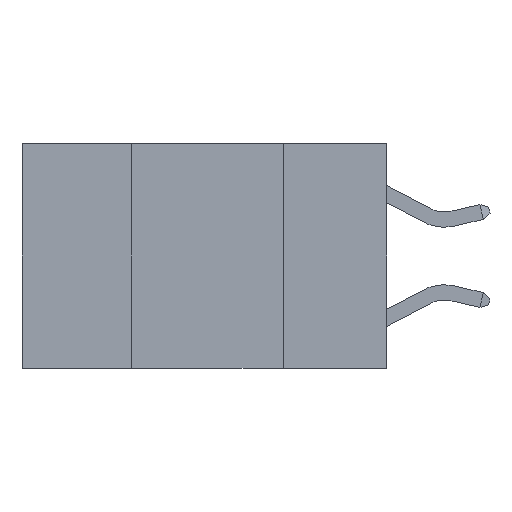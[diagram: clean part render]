
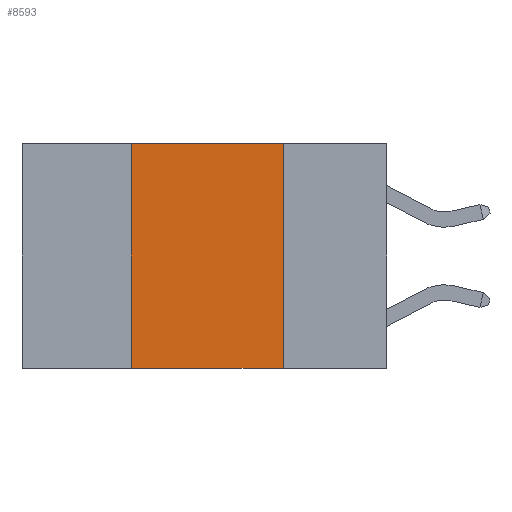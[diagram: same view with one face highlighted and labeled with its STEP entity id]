
A CAD part, left-side view. The second image highlights one B-rep face of the part: STEP entity #8593.
In plain terms, the highlighted planar face has unit normal (-1, 0, 0).
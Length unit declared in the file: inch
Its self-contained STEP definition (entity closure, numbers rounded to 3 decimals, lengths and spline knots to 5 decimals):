
#255 = VECTOR ( 'NONE', #6862, 39.37008 ) ;
#387 = VERTEX_POINT ( 'NONE', #7089 ) ;
#912 = EDGE_CURVE ( 'NONE', #1188, #9660, #5066, .T. ) ;
#1188 = VERTEX_POINT ( 'NONE', #4482 ) ;
#1473 = DIRECTION ( 'NONE',  ( 1., 0., 0. ) ) ;
#2008 = EDGE_CURVE ( 'NONE', #1188, #387, #6338, .T. ) ;
#2725 = VERTEX_POINT ( 'NONE', #5043 ) ;
#2930 = ORIENTED_EDGE ( 'NONE', *, *, #2008, .T. ) ;
#3427 = EDGE_CURVE ( 'NONE', #2725, #387, #4746, .T. ) ;
#3689 = LINE ( 'NONE', #4263, #4199 ) ;
#3884 = AXIS2_PLACEMENT_3D ( 'NONE', #6503, #1473, #7309 ) ;
#4199 = VECTOR ( 'NONE', #9939, 39.37008 ) ;
#4263 = CARTESIAN_POINT ( 'NONE',  ( 0., 0.6, 0. ) ) ;
#4283 = FACE_OUTER_BOUND ( 'NONE', #7953, .T. ) ;
#4482 = CARTESIAN_POINT ( 'NONE',  ( 0., 0.42, -0.37 ) ) ;
#4746 = LINE ( 'NONE', #7647, #255 ) ;
#5043 = CARTESIAN_POINT ( 'NONE',  ( 0., 0.17, 0. ) ) ;
#5066 = LINE ( 'NONE', #9829, #6742 ) ;
#5338 = ORIENTED_EDGE ( 'NONE', *, *, #912, .F. ) ;
#5722 = EDGE_CURVE ( 'NONE', #9660, #2725, #3689, .T. ) ;
#6338 = LINE ( 'NONE', #7128, #10356 ) ;
#6503 = CARTESIAN_POINT ( 'NONE',  ( 0., 0.6, 0. ) ) ;
#6742 = VECTOR ( 'NONE', #9778, 39.37008 ) ;
#6845 = ORIENTED_EDGE ( 'NONE', *, *, #5722, .F. ) ;
#6862 = DIRECTION ( 'NONE',  ( 0., 0., -1. ) ) ;
#7089 = CARTESIAN_POINT ( 'NONE',  ( 0., 0.17, -0.37 ) ) ;
#7128 = CARTESIAN_POINT ( 'NONE',  ( 0., 0.6, -0.37 ) ) ;
#7274 = PLANE ( 'NONE',  #3884 ) ;
#7309 = DIRECTION ( 'NONE',  ( 0., 0., -1. ) ) ;
#7351 = DIRECTION ( 'NONE',  ( 0., -1., 0. ) ) ;
#7647 = CARTESIAN_POINT ( 'NONE',  ( 0., 0.17, 0. ) ) ;
#7704 = CARTESIAN_POINT ( 'NONE',  ( 0., 0.42, 0. ) ) ;
#7953 = EDGE_LOOP ( 'NONE', ( #10040, #6845, #5338, #2930 ) ) ;
#8593 = ADVANCED_FACE ( 'NONE', ( #4283 ), #7274, .F. ) ;
#9660 = VERTEX_POINT ( 'NONE', #7704 ) ;
#9778 = DIRECTION ( 'NONE',  ( 0., 0., 1. ) ) ;
#9829 = CARTESIAN_POINT ( 'NONE',  ( 0., 0.42, 0. ) ) ;
#9939 = DIRECTION ( 'NONE',  ( 0., -1., 0. ) ) ;
#10040 = ORIENTED_EDGE ( 'NONE', *, *, #3427, .F. ) ;
#10356 = VECTOR ( 'NONE', #7351, 39.37008 ) ;
